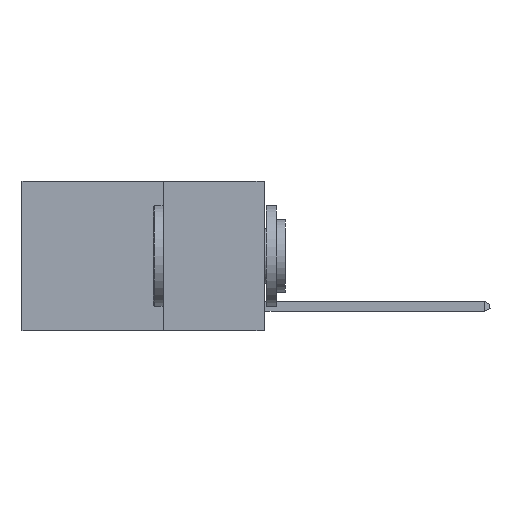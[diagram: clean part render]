
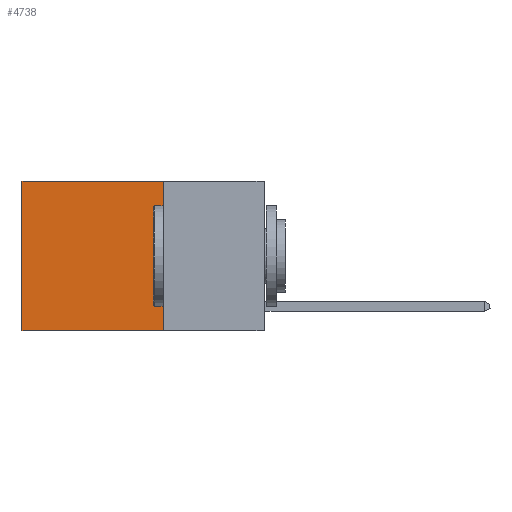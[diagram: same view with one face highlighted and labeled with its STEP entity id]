
A CAD part, left-side view. The second image highlights one B-rep face of the part: STEP entity #4738.
In plain terms, the highlighted planar face has unit normal (-1, 0, 0).
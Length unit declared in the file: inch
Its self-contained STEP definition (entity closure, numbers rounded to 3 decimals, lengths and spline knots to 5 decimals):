
#375 = VERTEX_POINT ( 'NONE', #17815 ) ;
#1986 = VECTOR ( 'NONE', #5244, 39.37008 ) ;
#2451 = DIRECTION ( 'NONE',  ( 0., 1., 0. ) ) ;
#4210 = VERTEX_POINT ( 'NONE', #9429 ) ;
#4248 = CARTESIAN_POINT ( 'NONE',  ( 0.2625, 0.6, -0.37 ) ) ;
#4709 = LINE ( 'NONE', #13424, #8881 ) ;
#4732 = CARTESIAN_POINT ( 'NONE',  ( 0.2625, 0.6, 0. ) ) ;
#4738 = ADVANCED_FACE ( 'NONE', ( #9669 ), #15414, .F. ) ;
#4822 = VERTEX_POINT ( 'NONE', #4732 ) ;
#5244 = DIRECTION ( 'NONE',  ( 0., 0., -1. ) ) ;
#5594 = EDGE_LOOP ( 'NONE', ( #14525, #18248, #13240, #9494 ) ) ;
#5699 = EDGE_CURVE ( 'NONE', #4210, #375, #6185, .T. ) ;
#6040 = CARTESIAN_POINT ( 'NONE',  ( 0.2625, 0.25, 0. ) ) ;
#6185 = LINE ( 'NONE', #14618, #1986 ) ;
#7614 = DIRECTION ( 'NONE',  ( 0., 0., -1. ) ) ;
#7668 = DIRECTION ( 'NONE',  ( 0., 1., 0. ) ) ;
#8630 = VECTOR ( 'NONE', #7668, 39.37008 ) ;
#8881 = VECTOR ( 'NONE', #2451, 39.37008 ) ;
#9429 = CARTESIAN_POINT ( 'NONE',  ( 0.2625, 0.25, 0. ) ) ;
#9494 = ORIENTED_EDGE ( 'NONE', *, *, #16245, .T. ) ;
#9669 = FACE_OUTER_BOUND ( 'NONE', #5594, .T. ) ;
#13240 = ORIENTED_EDGE ( 'NONE', *, *, #5699, .F. ) ;
#13424 = CARTESIAN_POINT ( 'NONE',  ( 0.2625, 0.25, 0. ) ) ;
#13951 = CARTESIAN_POINT ( 'NONE',  ( 0.2625, 0.25, -0.37 ) ) ;
#14287 = CARTESIAN_POINT ( 'NONE',  ( 0.2625, 0.6, 0. ) ) ;
#14525 = ORIENTED_EDGE ( 'NONE', *, *, #19534, .T. ) ;
#14618 = CARTESIAN_POINT ( 'NONE',  ( 0.2625, 0.25, 0. ) ) ;
#14846 = VERTEX_POINT ( 'NONE', #4248 ) ;
#15414 = PLANE ( 'NONE',  #16065 ) ;
#15972 = LINE ( 'NONE', #14287, #19195 ) ;
#16065 = AXIS2_PLACEMENT_3D ( 'NONE', #6040, #17021, #7614 ) ;
#16245 = EDGE_CURVE ( 'NONE', #4210, #4822, #4709, .T. ) ;
#16462 = LINE ( 'NONE', #13951, #8630 ) ;
#16506 = EDGE_CURVE ( 'NONE', #375, #14846, #16462, .T. ) ;
#17021 = DIRECTION ( 'NONE',  ( 1., 0., 0. ) ) ;
#17815 = CARTESIAN_POINT ( 'NONE',  ( 0.2625, 0.25, -0.37 ) ) ;
#18248 = ORIENTED_EDGE ( 'NONE', *, *, #16506, .F. ) ;
#19056 = DIRECTION ( 'NONE',  ( 0., 0., -1. ) ) ;
#19195 = VECTOR ( 'NONE', #19056, 39.37008 ) ;
#19534 = EDGE_CURVE ( 'NONE', #4822, #14846, #15972, .T. ) ;
